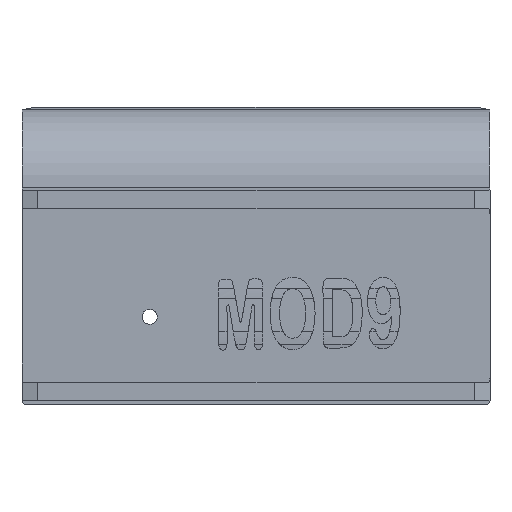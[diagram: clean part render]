
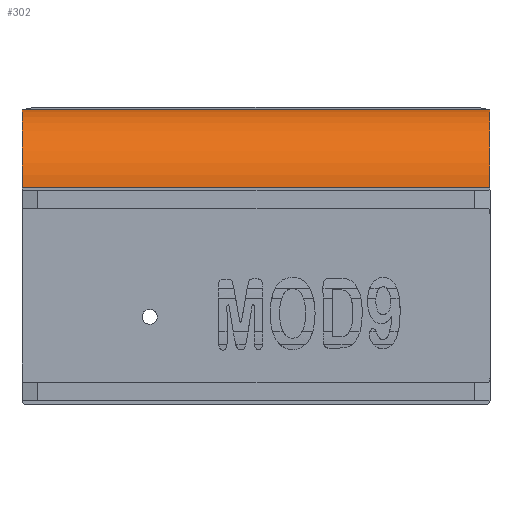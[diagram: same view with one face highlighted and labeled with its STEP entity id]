
A CAD part, top view. The second image highlights one B-rep face of the part: STEP entity #302.
In plain terms, the highlighted cylindrical face has radius 13 mm (diameter 26 mm), a partial arc.
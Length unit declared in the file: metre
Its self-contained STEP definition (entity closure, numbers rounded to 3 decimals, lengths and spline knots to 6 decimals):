
#302=ADVANCED_FACE('0:55584',(#867),#868,.T.);
#867=FACE_OUTER_BOUND('',#2860,.T.);
#868=CYLINDRICAL_SURFACE('',#2861,0.013);
#2860=EDGE_LOOP('',(#4808,#4809,#4810,#4811));
#2861=AXIS2_PLACEMENT_3D('',#4812,#4813,#4814);
#4808=ORIENTED_EDGE('',*,*,#6043,.F.);
#4809=ORIENTED_EDGE('',*,*,#6056,.T.);
#4810=ORIENTED_EDGE('',*,*,#6055,.T.);
#4811=ORIENTED_EDGE('',*,*,#5416,.F.);
#4812=CARTESIAN_POINT('',(-0.020295,0.047895,0.000681));
#4813=DIRECTION('',(-1.0,0.,0.));
#4814=DIRECTION('',(0.,0.,1.0));
#5416=EDGE_CURVE('0:55920',#6428,#6430,#6431,.T.);
#6043=EDGE_CURVE('0:57843',#7457,#6428,#7459,.T.);
#6055=EDGE_CURVE('0:57885',#7471,#6430,#7473,.F.);
#6056=EDGE_CURVE('0:57888',#7457,#7471,#7474,.T.);
#6428=VERTEX_POINT('',#8056);
#6430=VERTEX_POINT('',#8059);
#6431=CIRCLE('',#8060,0.013);
#7457=VERTEX_POINT('',#11152);
#7459=LINE('',#11155,#11156);
#7471=VERTEX_POINT('',#11177);
#7473=LINE('',#11180,#11181);
#7474=CIRCLE('',#11182,0.013);
#8056=CARTESIAN_POINT('',(-0.020295,0.060808,0.002181));
#8059=CARTESIAN_POINT('',(-0.020295,0.047907,0.013681));
#8060=AXIS2_PLACEMENT_3D('',#11647,#11648,#11649);
#11152=CARTESIAN_POINT('',(-0.097484,0.060808,0.002181));
#11155=CARTESIAN_POINT('',(-0.020295,0.060808,0.002181));
#11156=VECTOR('',#12112,0.077189);
#11177=CARTESIAN_POINT('',(-0.097484,0.047907,0.013681));
#11180=CARTESIAN_POINT('',(-0.020295,0.047907,0.013681));
#11181=VECTOR('',#12126,0.077189);
#11182=AXIS2_PLACEMENT_3D('',#12127,#12128,#12129);
#11647=CARTESIAN_POINT('',(-0.020295,0.047895,0.000681));
#11648=DIRECTION('',(1.0,0.,0.));
#11649=DIRECTION('',(0.,0.,1.0));
#12112=DIRECTION('',(1.0,0.,0.));
#12126=DIRECTION('',(-1.0,0.,0.));
#12127=CARTESIAN_POINT('',(-0.097484,0.047895,0.000681));
#12128=DIRECTION('',(1.0,0.,0.));
#12129=DIRECTION('',(0.,0.,1.0));
